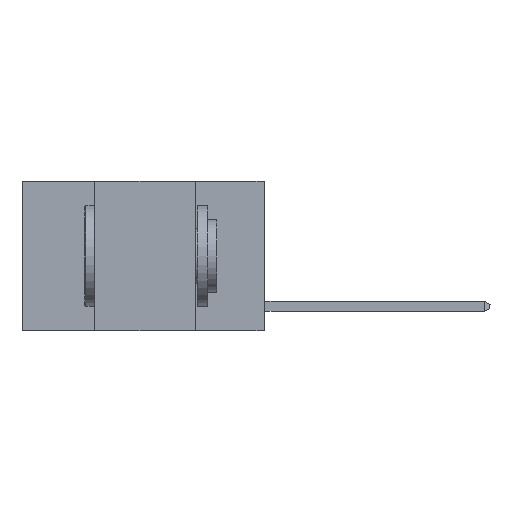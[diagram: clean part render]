
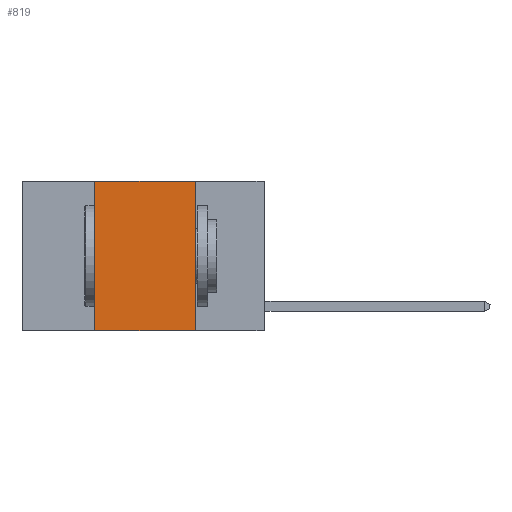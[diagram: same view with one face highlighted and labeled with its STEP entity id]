
A CAD part, left-side view. The second image highlights one B-rep face of the part: STEP entity #819.
In plain terms, the highlighted planar face has unit normal (-1, 0, 0).
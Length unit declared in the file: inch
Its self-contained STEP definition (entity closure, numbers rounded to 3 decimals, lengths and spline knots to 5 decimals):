
#22 = EDGE_LOOP ( 'NONE', ( #8265, #7962, #14067, #4208 ) ) ;
#51 = DIRECTION ( 'NONE',  ( 0., 0., -1. ) ) ;
#481 = CARTESIAN_POINT ( 'NONE',  ( 0., 0.17, 0. ) ) ;
#517 = LINE ( 'NONE', #6533, #6713 ) ;
#697 = DIRECTION ( 'NONE',  ( 0., 0., 1. ) ) ;
#819 = ADVANCED_FACE ( 'NONE', ( #8951 ), #11349, .F. ) ;
#833 = VERTEX_POINT ( 'NONE', #8932 ) ;
#2988 = EDGE_CURVE ( 'NONE', #833, #14722, #6502, .T. ) ;
#3293 = CARTESIAN_POINT ( 'NONE',  ( 0., 0.6, 0. ) ) ;
#3388 = VERTEX_POINT ( 'NONE', #481 ) ;
#4208 = ORIENTED_EDGE ( 'NONE', *, *, #2988, .T. ) ;
#5878 = CARTESIAN_POINT ( 'NONE',  ( 0., 0.17, 0. ) ) ;
#6502 = LINE ( 'NONE', #7504, #12395 ) ;
#6533 = CARTESIAN_POINT ( 'NONE',  ( 0., 0.42, 0. ) ) ;
#6544 = DIRECTION ( 'NONE',  ( 0., 0., -1. ) ) ;
#6713 = VECTOR ( 'NONE', #697, 39.37008 ) ;
#7504 = CARTESIAN_POINT ( 'NONE',  ( 0., 0.6, -0.37 ) ) ;
#7683 = DIRECTION ( 'NONE',  ( 0., -1., 0. ) ) ;
#7754 = LINE ( 'NONE', #5878, #10494 ) ;
#7962 = ORIENTED_EDGE ( 'NONE', *, *, #14890, .F. ) ;
#8265 = ORIENTED_EDGE ( 'NONE', *, *, #13089, .F. ) ;
#8932 = CARTESIAN_POINT ( 'NONE',  ( 0., 0.42, -0.37 ) ) ;
#8951 = FACE_OUTER_BOUND ( 'NONE', #22, .T. ) ;
#9345 = VECTOR ( 'NONE', #10315, 39.37008 ) ;
#10003 = CARTESIAN_POINT ( 'NONE',  ( 0., 0.17, -0.37 ) ) ;
#10315 = DIRECTION ( 'NONE',  ( 0., -1., 0. ) ) ;
#10360 = EDGE_CURVE ( 'NONE', #833, #13221, #517, .T. ) ;
#10494 = VECTOR ( 'NONE', #51, 39.37008 ) ;
#11100 = DIRECTION ( 'NONE',  ( 1., 0., 0. ) ) ;
#11344 = CARTESIAN_POINT ( 'NONE',  ( 0., 0.6, 0. ) ) ;
#11349 = PLANE ( 'NONE',  #13793 ) ;
#12395 = VECTOR ( 'NONE', #7683, 39.37008 ) ;
#12862 = LINE ( 'NONE', #3293, #9345 ) ;
#13089 = EDGE_CURVE ( 'NONE', #3388, #14722, #7754, .T. ) ;
#13137 = CARTESIAN_POINT ( 'NONE',  ( 0., 0.42, 0. ) ) ;
#13221 = VERTEX_POINT ( 'NONE', #13137 ) ;
#13793 = AXIS2_PLACEMENT_3D ( 'NONE', #11344, #11100, #6544 ) ;
#14067 = ORIENTED_EDGE ( 'NONE', *, *, #10360, .F. ) ;
#14722 = VERTEX_POINT ( 'NONE', #10003 ) ;
#14890 = EDGE_CURVE ( 'NONE', #13221, #3388, #12862, .T. ) ;
